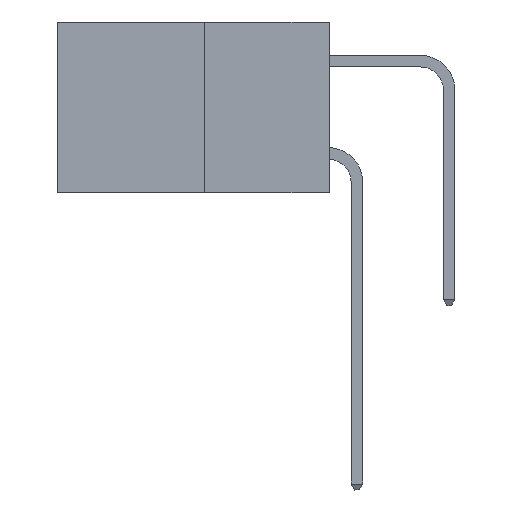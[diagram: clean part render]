
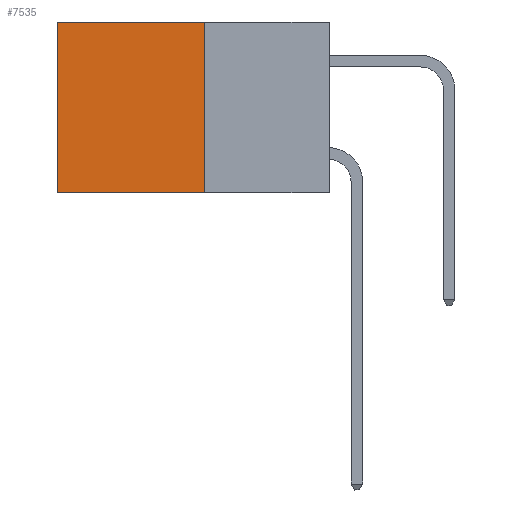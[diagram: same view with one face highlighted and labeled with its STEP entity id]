
A CAD part, left-side view. The second image highlights one B-rep face of the part: STEP entity #7535.
In plain terms, the highlighted planar face has unit normal (-1, 0, 0).
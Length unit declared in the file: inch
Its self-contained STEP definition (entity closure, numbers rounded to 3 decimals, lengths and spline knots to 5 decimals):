
#160 = EDGE_CURVE ( 'NONE', #8419, #6366, #11563, .T. ) ;
#349 = ORIENTED_EDGE ( 'NONE', *, *, #6177, .T. ) ;
#564 = VERTEX_POINT ( 'NONE', #5851 ) ;
#583 = EDGE_LOOP ( 'NONE', ( #349, #7779, #1234, #3405 ) ) ;
#1234 = ORIENTED_EDGE ( 'NONE', *, *, #2156, .F. ) ;
#1677 = EDGE_CURVE ( 'NONE', #4486, #564, #3317, .T. ) ;
#1712 = CARTESIAN_POINT ( 'NONE',  ( 0.277, 0.59, 0. ) ) ;
#2156 = EDGE_CURVE ( 'NONE', #8419, #4486, #5552, .T. ) ;
#2216 = DIRECTION ( 'NONE',  ( 0., 0., -1. ) ) ;
#2374 = LINE ( 'NONE', #6192, #11182 ) ;
#2477 = VECTOR ( 'NONE', #6671, 39.37008 ) ;
#2983 = VECTOR ( 'NONE', #6352, 39.37008 ) ;
#3317 = LINE ( 'NONE', #9306, #2983 ) ;
#3405 = ORIENTED_EDGE ( 'NONE', *, *, #160, .T. ) ;
#4486 = VERTEX_POINT ( 'NONE', #9319 ) ;
#5096 = CARTESIAN_POINT ( 'NONE',  ( 0.277, 0.27, -0.37 ) ) ;
#5552 = LINE ( 'NONE', #9258, #2477 ) ;
#5851 = CARTESIAN_POINT ( 'NONE',  ( 0.277, 0.59, -0.37 ) ) ;
#6177 = EDGE_CURVE ( 'NONE', #6366, #564, #2374, .T. ) ;
#6192 = CARTESIAN_POINT ( 'NONE',  ( 0.277, 0.59, -0.37 ) ) ;
#6352 = DIRECTION ( 'NONE',  ( 0., 1., 0. ) ) ;
#6366 = VERTEX_POINT ( 'NONE', #1712 ) ;
#6671 = DIRECTION ( 'NONE',  ( 0., 0., -1. ) ) ;
#7294 = AXIS2_PLACEMENT_3D ( 'NONE', #5096, #7478, #2216 ) ;
#7402 = PLANE ( 'NONE',  #7294 ) ;
#7478 = DIRECTION ( 'NONE',  ( 1., 0., 0. ) ) ;
#7535 = ADVANCED_FACE ( 'NONE', ( #10798 ), #7402, .F. ) ;
#7779 = ORIENTED_EDGE ( 'NONE', *, *, #1677, .F. ) ;
#8419 = VERTEX_POINT ( 'NONE', #11207 ) ;
#9258 = CARTESIAN_POINT ( 'NONE',  ( 0.277, 0.27, -0.37 ) ) ;
#9306 = CARTESIAN_POINT ( 'NONE',  ( 0.277, 0.27, -0.37 ) ) ;
#9319 = CARTESIAN_POINT ( 'NONE',  ( 0.277, 0.27, -0.37 ) ) ;
#10284 = DIRECTION ( 'NONE',  ( 0., 0., -1. ) ) ;
#10798 = FACE_OUTER_BOUND ( 'NONE', #583, .T. ) ;
#10995 = CARTESIAN_POINT ( 'NONE',  ( 0.277, 0.27, 0. ) ) ;
#11015 = DIRECTION ( 'NONE',  ( 0., 1., 0. ) ) ;
#11182 = VECTOR ( 'NONE', #10284, 39.37008 ) ;
#11207 = CARTESIAN_POINT ( 'NONE',  ( 0.277, 0.27, 0. ) ) ;
#11330 = VECTOR ( 'NONE', #11015, 39.37008 ) ;
#11563 = LINE ( 'NONE', #10995, #11330 ) ;
